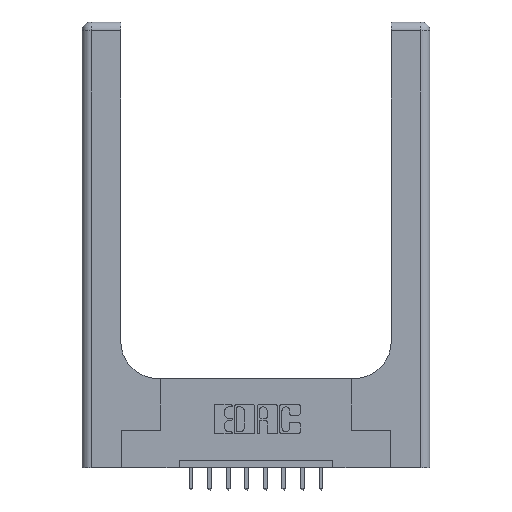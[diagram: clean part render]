
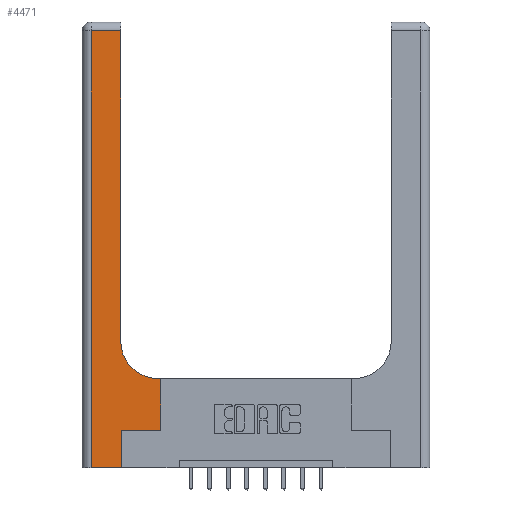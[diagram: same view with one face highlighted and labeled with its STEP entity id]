
A CAD part, top view. The second image highlights one B-rep face of the part: STEP entity #4471.
In plain terms, the highlighted planar face has unit normal (0, 0, 1).
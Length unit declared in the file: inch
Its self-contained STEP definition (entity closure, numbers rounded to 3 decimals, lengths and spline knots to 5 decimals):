
#273 = CARTESIAN_POINT ( 'NONE',  ( 0.06, 2.94, 0.37 ) ) ;
#361 = PLANE ( 'NONE',  #10439 ) ;
#441 = FACE_OUTER_BOUND ( 'NONE', #2237, .T. ) ;
#456 = CARTESIAN_POINT ( 'NONE',  ( 0.06, 3., 0.37 ) ) ;
#851 = VERTEX_POINT ( 'NONE', #14127 ) ;
#1053 = LINE ( 'NONE', #10382, #13323 ) ;
#1206 = DIRECTION ( 'NONE',  ( 0., 1., 0. ) ) ;
#1255 = DIRECTION ( 'NONE',  ( 1., 0., 0. ) ) ;
#1623 = VERTEX_POINT ( 'NONE', #273 ) ;
#1826 = DIRECTION ( 'NONE',  ( -1., 0., 0. ) ) ;
#2237 = EDGE_LOOP ( 'NONE', ( #6169, #13462, #12691, #5627, #4194, #10381, #12762, #3961, #6347 ) ) ;
#2254 = LINE ( 'NONE', #3542, #5423 ) ;
#2339 = VECTOR ( 'NONE', #4432, 39.37008 ) ;
#2362 = CARTESIAN_POINT ( 'NONE',  ( 0.51, 0.85, 0.37 ) ) ;
#2460 = CARTESIAN_POINT ( 'NONE',  ( 0.265, 0.25, 0.37 ) ) ;
#2467 = CARTESIAN_POINT ( 'NONE',  ( 0.26, 0.6, 0.37 ) ) ;
#2556 = EDGE_CURVE ( 'NONE', #851, #7371, #11515, .T. ) ;
#3088 = EDGE_CURVE ( 'NONE', #7890, #13903, #14252, .T. ) ;
#3326 = CARTESIAN_POINT ( 'NONE',  ( 0.528, 0.25, 0.37 ) ) ;
#3542 = CARTESIAN_POINT ( 'NONE',  ( 0., 0., 0.37 ) ) ;
#3598 = LINE ( 'NONE', #14274, #15097 ) ;
#3735 = DIRECTION ( 'NONE',  ( 1., 0., 0. ) ) ;
#3921 = EDGE_CURVE ( 'NONE', #4603, #9623, #3598, .T. ) ;
#3961 = ORIENTED_EDGE ( 'NONE', *, *, #13155, .T. ) ;
#4194 = ORIENTED_EDGE ( 'NONE', *, *, #2556, .T. ) ;
#4269 = DIRECTION ( 'NONE',  ( -1., 0., 0. ) ) ;
#4349 = VERTEX_POINT ( 'NONE', #4721 ) ;
#4432 = DIRECTION ( 'NONE',  ( 0., 1., 0. ) ) ;
#4471 = ADVANCED_FACE ( 'NONE', ( #441 ), #361, .F. ) ;
#4527 = VECTOR ( 'NONE', #1206, 39.37008 ) ;
#4603 = VERTEX_POINT ( 'NONE', #3326 ) ;
#4721 = CARTESIAN_POINT ( 'NONE',  ( 0.51, 0.6, 0.37 ) ) ;
#5311 = EDGE_CURVE ( 'NONE', #4349, #7890, #12209, .T. ) ;
#5423 = VECTOR ( 'NONE', #1255, 39.37008 ) ;
#5627 = ORIENTED_EDGE ( 'NONE', *, *, #11552, .T. ) ;
#5966 = CARTESIAN_POINT ( 'NONE',  ( 0.265, 0.25, 0.37 ) ) ;
#6169 = ORIENTED_EDGE ( 'NONE', *, *, #3088, .T. ) ;
#6185 = VECTOR ( 'NONE', #12269, 39.37008 ) ;
#6278 = EDGE_CURVE ( 'NONE', #7371, #4603, #6408, .T. ) ;
#6305 = AXIS2_PLACEMENT_3D ( 'NONE', #2362, #11729, #3735 ) ;
#6347 = ORIENTED_EDGE ( 'NONE', *, *, #5311, .T. ) ;
#6408 = LINE ( 'NONE', #5966, #14381 ) ;
#7371 = VERTEX_POINT ( 'NONE', #2460 ) ;
#7494 = DIRECTION ( 'NONE',  ( 1., 0., 0. ) ) ;
#7890 = VERTEX_POINT ( 'NONE', #14781 ) ;
#8063 = CARTESIAN_POINT ( 'NONE',  ( 0.265, 0., 0.37 ) ) ;
#8719 = CARTESIAN_POINT ( 'NONE',  ( 0., 3., 0.37 ) ) ;
#9623 = VERTEX_POINT ( 'NONE', #14182 ) ;
#10381 = ORIENTED_EDGE ( 'NONE', *, *, #6278, .T. ) ;
#10382 = CARTESIAN_POINT ( 'NONE',  ( 0., 2.94, 0.37 ) ) ;
#10439 = AXIS2_PLACEMENT_3D ( 'NONE', #8719, #11102, #1826 ) ;
#10863 = CARTESIAN_POINT ( 'NONE',  ( 0.26, 2.94, 0.37 ) ) ;
#11102 = DIRECTION ( 'NONE',  ( 0., 0., -1. ) ) ;
#11116 = LINE ( 'NONE', #456, #6185 ) ;
#11515 = LINE ( 'NONE', #8063, #2339 ) ;
#11552 = EDGE_CURVE ( 'NONE', #14940, #851, #2254, .T. ) ;
#11559 = VECTOR ( 'NONE', #12826, 39.37008 ) ;
#11729 = DIRECTION ( 'NONE',  ( 0., 0., -1. ) ) ;
#11974 = DIRECTION ( 'NONE',  ( 0., 1., 0. ) ) ;
#12209 = CIRCLE ( 'NONE', #6305, 0.25 ) ;
#12269 = DIRECTION ( 'NONE',  ( 0., -1., 0. ) ) ;
#12691 = ORIENTED_EDGE ( 'NONE', *, *, #14806, .T. ) ;
#12762 = ORIENTED_EDGE ( 'NONE', *, *, #3921, .T. ) ;
#12826 = DIRECTION ( 'NONE',  ( -1., 0., 0. ) ) ;
#12955 = CARTESIAN_POINT ( 'NONE',  ( 0.26, 3., 0.37 ) ) ;
#13155 = EDGE_CURVE ( 'NONE', #9623, #4349, #13981, .T. ) ;
#13323 = VECTOR ( 'NONE', #4269, 39.37008 ) ;
#13462 = ORIENTED_EDGE ( 'NONE', *, *, #14997, .T. ) ;
#13652 = CARTESIAN_POINT ( 'NONE',  ( 0.06, 0., 0.37 ) ) ;
#13903 = VERTEX_POINT ( 'NONE', #10863 ) ;
#13981 = LINE ( 'NONE', #2467, #11559 ) ;
#14127 = CARTESIAN_POINT ( 'NONE',  ( 0.265, 0., 0.37 ) ) ;
#14182 = CARTESIAN_POINT ( 'NONE',  ( 0.528, 0.6, 0.37 ) ) ;
#14252 = LINE ( 'NONE', #12955, #4527 ) ;
#14274 = CARTESIAN_POINT ( 'NONE',  ( 0.528, 0.25, 0.37 ) ) ;
#14381 = VECTOR ( 'NONE', #7494, 39.37008 ) ;
#14781 = CARTESIAN_POINT ( 'NONE',  ( 0.26, 0.85, 0.37 ) ) ;
#14806 = EDGE_CURVE ( 'NONE', #1623, #14940, #11116, .T. ) ;
#14940 = VERTEX_POINT ( 'NONE', #13652 ) ;
#14997 = EDGE_CURVE ( 'NONE', #13903, #1623, #1053, .T. ) ;
#15097 = VECTOR ( 'NONE', #11974, 39.37008 ) ;
